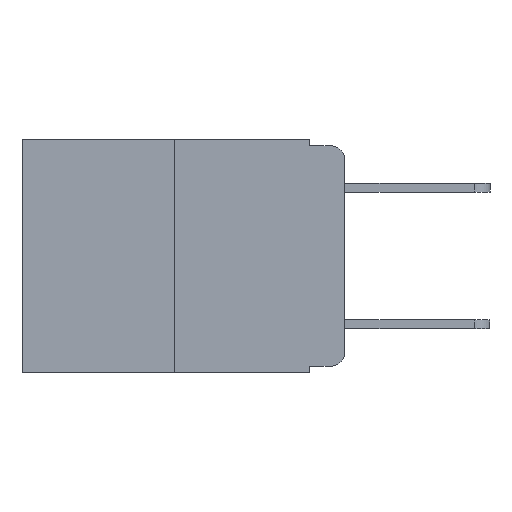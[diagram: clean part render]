
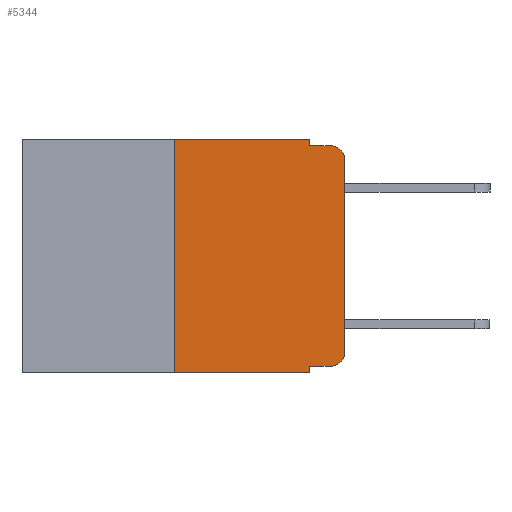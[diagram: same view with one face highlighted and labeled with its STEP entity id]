
A CAD part, left-side view. The second image highlights one B-rep face of the part: STEP entity #5344.
In plain terms, the highlighted planar face has unit normal (-1, 0, 0).
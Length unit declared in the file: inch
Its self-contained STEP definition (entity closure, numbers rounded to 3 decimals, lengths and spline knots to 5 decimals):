
#24 = VERTEX_POINT ( 'NONE', #8485 ) ;
#191 = ORIENTED_EDGE ( 'NONE', *, *, #2380, .F. ) ;
#347 = VERTEX_POINT ( 'NONE', #6358 ) ;
#404 = VERTEX_POINT ( 'NONE', #1634 ) ;
#415 = EDGE_CURVE ( 'NONE', #11359, #1471, #8568, .T. ) ;
#438 = ORIENTED_EDGE ( 'NONE', *, *, #11109, .F. ) ;
#491 = ORIENTED_EDGE ( 'NONE', *, *, #5516, .T. ) ;
#844 = LINE ( 'NONE', #1845, #5703 ) ;
#885 = VERTEX_POINT ( 'NONE', #3484 ) ;
#1434 = ORIENTED_EDGE ( 'NONE', *, *, #7433, .F. ) ;
#1471 = VERTEX_POINT ( 'NONE', #5268 ) ;
#1546 = VERTEX_POINT ( 'NONE', #3446 ) ;
#1627 = AXIS2_PLACEMENT_3D ( 'NONE', #5381, #11200, #6289 ) ;
#1634 = CARTESIAN_POINT ( 'NONE',  ( 0., 0.051, 0. ) ) ;
#1685 = EDGE_CURVE ( 'NONE', #5322, #347, #6643, .T. ) ;
#1833 = DIRECTION ( 'NONE',  ( 1., 0., 0. ) ) ;
#1845 = CARTESIAN_POINT ( 'NONE',  ( 0., 0.473, -0.343 ) ) ;
#2076 = DIRECTION ( 'NONE',  ( 0., -1., 0. ) ) ;
#2137 = VECTOR ( 'NONE', #6661, 39.37008 ) ;
#2354 = VERTEX_POINT ( 'NONE', #8026 ) ;
#2380 = EDGE_CURVE ( 'NONE', #1471, #404, #3733, .T. ) ;
#2432 = LINE ( 'NONE', #2642, #11267 ) ;
#2603 = LINE ( 'NONE', #8458, #7087 ) ;
#2642 = CARTESIAN_POINT ( 'NONE',  ( 0., 0.051, -0.01 ) ) ;
#2932 = CARTESIAN_POINT ( 'NONE',  ( 0., 0.473, 0. ) ) ;
#2980 = ORIENTED_EDGE ( 'NONE', *, *, #10980, .T. ) ;
#3008 = VECTOR ( 'NONE', #6883, 39.37008 ) ;
#3114 = DIRECTION ( 'NONE',  ( -1., 0., 0. ) ) ;
#3446 = CARTESIAN_POINT ( 'NONE',  ( 0., 0.051, -0.333 ) ) ;
#3484 = CARTESIAN_POINT ( 'NONE',  ( 0., 0.051, -0.343 ) ) ;
#3501 = ORIENTED_EDGE ( 'NONE', *, *, #10118, .F. ) ;
#3733 = LINE ( 'NONE', #2932, #10051 ) ;
#3778 = PLANE ( 'NONE',  #6561 ) ;
#3908 = VECTOR ( 'NONE', #8797, 39.37008 ) ;
#3999 = CARTESIAN_POINT ( 'NONE',  ( 0., 0.051, -0.333 ) ) ;
#5189 = AXIS2_PLACEMENT_3D ( 'NONE', #8397, #3114, #9250 ) ;
#5268 = CARTESIAN_POINT ( 'NONE',  ( 0., 0.25, 0. ) ) ;
#5322 = VERTEX_POINT ( 'NONE', #11320 ) ;
#5344 = ADVANCED_FACE ( 'NONE', ( #10445 ), #3778, .F. ) ;
#5381 = CARTESIAN_POINT ( 'NONE',  ( 0., 0.02, -0.03 ) ) ;
#5390 = CIRCLE ( 'NONE', #1627, 0.02 ) ;
#5516 = EDGE_CURVE ( 'NONE', #1546, #2354, #6954, .T. ) ;
#5541 = ORIENTED_EDGE ( 'NONE', *, *, #415, .F. ) ;
#5557 = DIRECTION ( 'NONE',  ( 0., -1., 0. ) ) ;
#5579 = ORIENTED_EDGE ( 'NONE', *, *, #10373, .T. ) ;
#5703 = VECTOR ( 'NONE', #5557, 39.37008 ) ;
#6168 = ORIENTED_EDGE ( 'NONE', *, *, #10746, .T. ) ;
#6289 = DIRECTION ( 'NONE',  ( 0., 0., -1. ) ) ;
#6358 = CARTESIAN_POINT ( 'NONE',  ( 0., 0., -0.03 ) ) ;
#6561 = AXIS2_PLACEMENT_3D ( 'NONE', #11348, #1833, #8180 ) ;
#6567 = CARTESIAN_POINT ( 'NONE',  ( 0., 0.02, -0.01 ) ) ;
#6643 = LINE ( 'NONE', #9608, #10784 ) ;
#6661 = DIRECTION ( 'NONE',  ( 0., -1., 0. ) ) ;
#6883 = DIRECTION ( 'NONE',  ( 0., 0., -1. ) ) ;
#6954 = LINE ( 'NONE', #3999, #2137 ) ;
#7087 = VECTOR ( 'NONE', #9295, 39.37008 ) ;
#7433 = EDGE_CURVE ( 'NONE', #404, #24, #2603, .T. ) ;
#7710 = LINE ( 'NONE', #9424, #3008 ) ;
#8026 = CARTESIAN_POINT ( 'NONE',  ( 0., 0.02, -0.333 ) ) ;
#8180 = DIRECTION ( 'NONE',  ( 0., 0., -1. ) ) ;
#8397 = CARTESIAN_POINT ( 'NONE',  ( 0., 0.02, -0.313 ) ) ;
#8458 = CARTESIAN_POINT ( 'NONE',  ( 0., 0.051, 0. ) ) ;
#8485 = CARTESIAN_POINT ( 'NONE',  ( 0., 0.051, -0.01 ) ) ;
#8568 = LINE ( 'NONE', #8908, #3908 ) ;
#8797 = DIRECTION ( 'NONE',  ( 0., 0., 1. ) ) ;
#8908 = CARTESIAN_POINT ( 'NONE',  ( 0., 0.25, 0. ) ) ;
#9235 = ORIENTED_EDGE ( 'NONE', *, *, #1685, .T. ) ;
#9244 = EDGE_LOOP ( 'NONE', ( #9235, #6168, #3501, #1434, #191, #5541, #5579, #438, #491, #2980 ) ) ;
#9250 = DIRECTION ( 'NONE',  ( 0., 0., -1. ) ) ;
#9295 = DIRECTION ( 'NONE',  ( 0., 0., -1. ) ) ;
#9424 = CARTESIAN_POINT ( 'NONE',  ( 0., 0.051, 0. ) ) ;
#9571 = CIRCLE ( 'NONE', #5189, 0.02 ) ;
#9608 = CARTESIAN_POINT ( 'NONE',  ( 0., 0., 0. ) ) ;
#10051 = VECTOR ( 'NONE', #2076, 39.37008 ) ;
#10118 = EDGE_CURVE ( 'NONE', #24, #10274, #2432, .T. ) ;
#10274 = VERTEX_POINT ( 'NONE', #6567 ) ;
#10373 = EDGE_CURVE ( 'NONE', #11359, #885, #844, .T. ) ;
#10445 = FACE_OUTER_BOUND ( 'NONE', #9244, .T. ) ;
#10542 = DIRECTION ( 'NONE',  ( 0., 0., 1. ) ) ;
#10562 = CARTESIAN_POINT ( 'NONE',  ( 0., 0.25, -0.343 ) ) ;
#10746 = EDGE_CURVE ( 'NONE', #347, #10274, #5390, .T. ) ;
#10784 = VECTOR ( 'NONE', #10542, 39.37008 ) ;
#10980 = EDGE_CURVE ( 'NONE', #2354, #5322, #9571, .T. ) ;
#11109 = EDGE_CURVE ( 'NONE', #1546, #885, #7710, .T. ) ;
#11151 = DIRECTION ( 'NONE',  ( 0., -1., 0. ) ) ;
#11200 = DIRECTION ( 'NONE',  ( -1., 0., 0. ) ) ;
#11267 = VECTOR ( 'NONE', #11151, 39.37008 ) ;
#11320 = CARTESIAN_POINT ( 'NONE',  ( 0., 0., -0.313 ) ) ;
#11348 = CARTESIAN_POINT ( 'NONE',  ( 0., 0.473, 0. ) ) ;
#11359 = VERTEX_POINT ( 'NONE', #10562 ) ;
